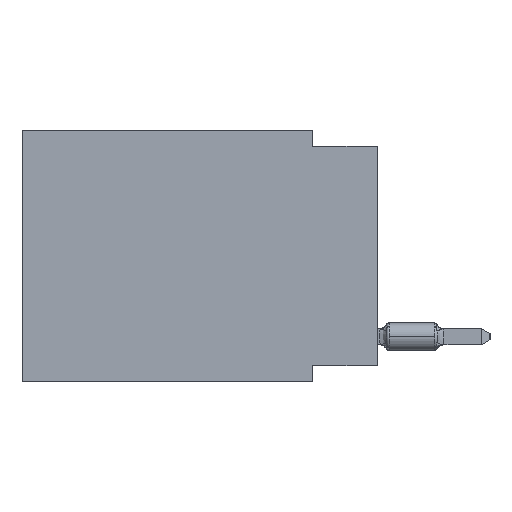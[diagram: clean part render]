
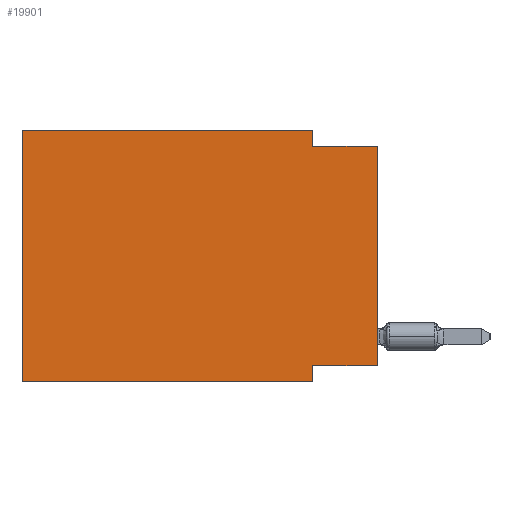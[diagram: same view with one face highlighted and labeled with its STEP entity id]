
A CAD part, left-side view. The second image highlights one B-rep face of the part: STEP entity #19901.
In plain terms, the highlighted planar face has unit normal (-1, 0, 0).
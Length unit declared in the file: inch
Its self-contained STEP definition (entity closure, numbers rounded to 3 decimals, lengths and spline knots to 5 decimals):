
#580 = AXIS2_PLACEMENT_3D ( 'NONE', #22927, #20900, #8848 ) ;
#609 = DIRECTION ( 'NONE',  ( 0., 0., 1. ) ) ;
#681 = PLANE ( 'NONE',  #580 ) ;
#947 = EDGE_CURVE ( 'NONE', #7053, #15619, #4613, .T. ) ;
#1197 = CARTESIAN_POINT ( 'NONE',  ( 0., 0.55, 0. ) ) ;
#1239 = CARTESIAN_POINT ( 'NONE',  ( 0., 0.55, 0. ) ) ;
#1474 = LINE ( 'NONE', #13383, #18030 ) ;
#1926 = CARTESIAN_POINT ( 'NONE',  ( 0., 0.1, 0. ) ) ;
#2159 = DIRECTION ( 'NONE',  ( 0., -1., 0. ) ) ;
#2207 = EDGE_CURVE ( 'NONE', #10270, #11562, #4145, .T. ) ;
#2630 = DIRECTION ( 'NONE',  ( 0., -1., 0. ) ) ;
#2770 = CARTESIAN_POINT ( 'NONE',  ( 0., 0.55, 0. ) ) ;
#4131 = EDGE_LOOP ( 'NONE', ( #11412, #23277, #17014, #23843, #23644, #16399, #24223, #10342 ) ) ;
#4145 = LINE ( 'NONE', #12310, #20579 ) ;
#4613 = LINE ( 'NONE', #18954, #10430 ) ;
#5088 = CARTESIAN_POINT ( 'NONE',  ( 0., 0.1, 0. ) ) ;
#5808 = CARTESIAN_POINT ( 'NONE',  ( 0., 0., -0.365 ) ) ;
#7053 = VERTEX_POINT ( 'NONE', #5808 ) ;
#7599 = VECTOR ( 'NONE', #21620, 39.37008 ) ;
#7790 = EDGE_CURVE ( 'NONE', #15765, #15619, #1474, .T. ) ;
#8848 = DIRECTION ( 'NONE',  ( 0., 0., -1. ) ) ;
#9400 = VECTOR ( 'NONE', #17539, 39.37008 ) ;
#9410 = DIRECTION ( 'NONE',  ( 0., 0., 1. ) ) ;
#10057 = CARTESIAN_POINT ( 'NONE',  ( 0., 0.1, -0.025 ) ) ;
#10218 = VECTOR ( 'NONE', #9410, 39.37008 ) ;
#10270 = VERTEX_POINT ( 'NONE', #23646 ) ;
#10342 = ORIENTED_EDGE ( 'NONE', *, *, #21361, .F. ) ;
#10430 = VECTOR ( 'NONE', #609, 39.37008 ) ;
#11412 = ORIENTED_EDGE ( 'NONE', *, *, #947, .T. ) ;
#11562 = VERTEX_POINT ( 'NONE', #18006 ) ;
#11826 = EDGE_CURVE ( 'NONE', #10270, #25013, #21332, .T. ) ;
#12003 = VERTEX_POINT ( 'NONE', #1926 ) ;
#12210 = EDGE_CURVE ( 'NONE', #12003, #15765, #19436, .T. ) ;
#12310 = CARTESIAN_POINT ( 'NONE',  ( 0., 0.55, -0.39 ) ) ;
#12467 = FACE_OUTER_BOUND ( 'NONE', #4131, .T. ) ;
#13383 = CARTESIAN_POINT ( 'NONE',  ( 0., 0., -0.025 ) ) ;
#14936 = LINE ( 'NONE', #2770, #20013 ) ;
#15619 = VERTEX_POINT ( 'NONE', #23604 ) ;
#15765 = VERTEX_POINT ( 'NONE', #10057 ) ;
#15982 = CARTESIAN_POINT ( 'NONE',  ( 0., 0., -0.365 ) ) ;
#16399 = ORIENTED_EDGE ( 'NONE', *, *, #2207, .T. ) ;
#17014 = ORIENTED_EDGE ( 'NONE', *, *, #12210, .F. ) ;
#17539 = DIRECTION ( 'NONE',  ( 0., 0., -1. ) ) ;
#17595 = CARTESIAN_POINT ( 'NONE',  ( 0., 0.1, -0.39 ) ) ;
#18006 = CARTESIAN_POINT ( 'NONE',  ( 0., 0.1, -0.39 ) ) ;
#18030 = VECTOR ( 'NONE', #25976, 39.37008 ) ;
#18954 = CARTESIAN_POINT ( 'NONE',  ( 0., 0., 0. ) ) ;
#19162 = VECTOR ( 'NONE', #24167, 39.37008 ) ;
#19436 = LINE ( 'NONE', #5088, #9400 ) ;
#19901 = ADVANCED_FACE ( 'NONE', ( #12467 ), #681, .F. ) ;
#20013 = VECTOR ( 'NONE', #2630, 39.37008 ) ;
#20039 = CARTESIAN_POINT ( 'NONE',  ( 0., 0.1, -0.365 ) ) ;
#20579 = VECTOR ( 'NONE', #2159, 39.37008 ) ;
#20900 = DIRECTION ( 'NONE',  ( 1., 0., 0. ) ) ;
#21332 = LINE ( 'NONE', #1239, #10218 ) ;
#21361 = EDGE_CURVE ( 'NONE', #7053, #23746, #26424, .T. ) ;
#21620 = DIRECTION ( 'NONE',  ( 0., 0., -1. ) ) ;
#22394 = LINE ( 'NONE', #17595, #7599 ) ;
#22816 = EDGE_CURVE ( 'NONE', #25013, #12003, #14936, .T. ) ;
#22927 = CARTESIAN_POINT ( 'NONE',  ( 0., 0.55, 0. ) ) ;
#22941 = EDGE_CURVE ( 'NONE', #23746, #11562, #22394, .T. ) ;
#23277 = ORIENTED_EDGE ( 'NONE', *, *, #7790, .F. ) ;
#23604 = CARTESIAN_POINT ( 'NONE',  ( 0., 0., -0.025 ) ) ;
#23644 = ORIENTED_EDGE ( 'NONE', *, *, #11826, .F. ) ;
#23646 = CARTESIAN_POINT ( 'NONE',  ( 0., 0.55, -0.39 ) ) ;
#23746 = VERTEX_POINT ( 'NONE', #20039 ) ;
#23843 = ORIENTED_EDGE ( 'NONE', *, *, #22816, .F. ) ;
#24167 = DIRECTION ( 'NONE',  ( 0., 1., 0. ) ) ;
#24223 = ORIENTED_EDGE ( 'NONE', *, *, #22941, .F. ) ;
#25013 = VERTEX_POINT ( 'NONE', #1197 ) ;
#25976 = DIRECTION ( 'NONE',  ( 0., -1., 0. ) ) ;
#26424 = LINE ( 'NONE', #15982, #19162 ) ;
